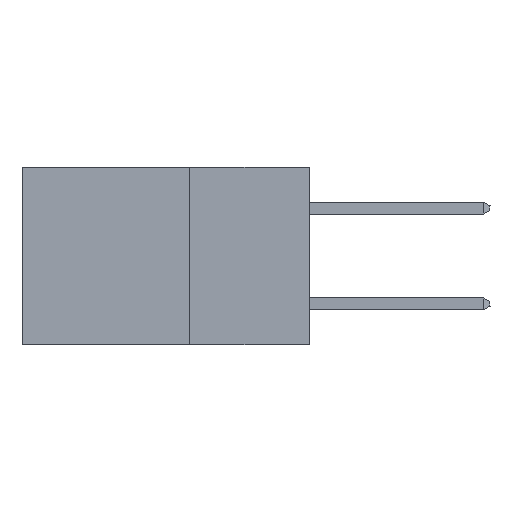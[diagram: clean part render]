
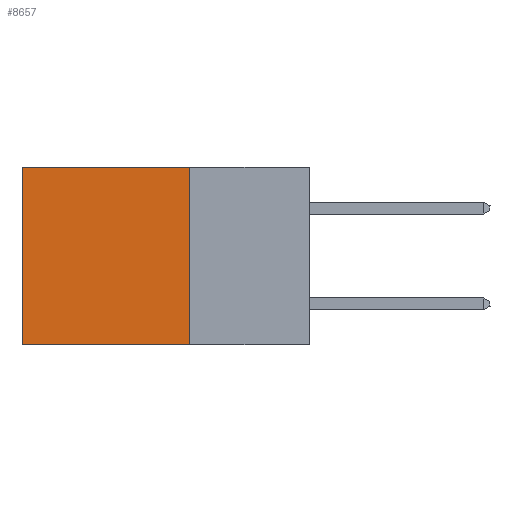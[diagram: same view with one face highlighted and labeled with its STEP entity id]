
A CAD part, left-side view. The second image highlights one B-rep face of the part: STEP entity #8657.
In plain terms, the highlighted planar face has unit normal (-1, 0, 0).
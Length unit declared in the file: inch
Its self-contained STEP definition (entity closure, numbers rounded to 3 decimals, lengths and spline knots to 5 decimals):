
#1060 = DIRECTION ( 'NONE',  ( 0., 1., 0. ) ) ;
#1374 = CARTESIAN_POINT ( 'NONE',  ( 0.2875, 0.25, -0.37 ) ) ;
#1828 = VECTOR ( 'NONE', #12287, 39.37008 ) ;
#1900 = CARTESIAN_POINT ( 'NONE',  ( 0.2875, 0.6, -0.37 ) ) ;
#3026 = CARTESIAN_POINT ( 'NONE',  ( 0.2875, 0.25, 0. ) ) ;
#3926 = VERTEX_POINT ( 'NONE', #17278 ) ;
#4363 = ORIENTED_EDGE ( 'NONE', *, *, #5215, .T. ) ;
#5124 = FACE_OUTER_BOUND ( 'NONE', #15097, .T. ) ;
#5215 = EDGE_CURVE ( 'NONE', #13371, #7720, #6733, .T. ) ;
#5445 = CARTESIAN_POINT ( 'NONE',  ( 0.2875, 0.6, 0. ) ) ;
#5970 = CARTESIAN_POINT ( 'NONE',  ( 0.2875, 0.6, 0. ) ) ;
#6553 = CARTESIAN_POINT ( 'NONE',  ( 0.2875, 0.25, -0.37 ) ) ;
#6733 = LINE ( 'NONE', #5445, #13678 ) ;
#6949 = CARTESIAN_POINT ( 'NONE',  ( 0.2875, 0.25, 0. ) ) ;
#7202 = VECTOR ( 'NONE', #1060, 39.37008 ) ;
#7720 = VERTEX_POINT ( 'NONE', #1900 ) ;
#8106 = VERTEX_POINT ( 'NONE', #1374 ) ;
#8268 = DIRECTION ( 'NONE',  ( 0., 0., -1. ) ) ;
#8657 = ADVANCED_FACE ( 'NONE', ( #5124 ), #14762, .F. ) ;
#9138 = ORIENTED_EDGE ( 'NONE', *, *, #10377, .T. ) ;
#9436 = EDGE_CURVE ( 'NONE', #8106, #7720, #17158, .T. ) ;
#10338 = AXIS2_PLACEMENT_3D ( 'NONE', #6949, #16045, #8268 ) ;
#10377 = EDGE_CURVE ( 'NONE', #3926, #13371, #16341, .T. ) ;
#10893 = DIRECTION ( 'NONE',  ( 0., 0., -1. ) ) ;
#12287 = DIRECTION ( 'NONE',  ( 0., 1., 0. ) ) ;
#13371 = VERTEX_POINT ( 'NONE', #5970 ) ;
#13440 = VECTOR ( 'NONE', #10893, 39.37008 ) ;
#13524 = CARTESIAN_POINT ( 'NONE',  ( 0.2875, 0.25, 0. ) ) ;
#13678 = VECTOR ( 'NONE', #17192, 39.37008 ) ;
#13866 = LINE ( 'NONE', #13524, #13440 ) ;
#14742 = ORIENTED_EDGE ( 'NONE', *, *, #15134, .F. ) ;
#14762 = PLANE ( 'NONE',  #10338 ) ;
#14922 = ORIENTED_EDGE ( 'NONE', *, *, #9436, .F. ) ;
#15097 = EDGE_LOOP ( 'NONE', ( #4363, #14922, #14742, #9138 ) ) ;
#15134 = EDGE_CURVE ( 'NONE', #3926, #8106, #13866, .T. ) ;
#16045 = DIRECTION ( 'NONE',  ( 1., 0., 0. ) ) ;
#16341 = LINE ( 'NONE', #3026, #1828 ) ;
#17158 = LINE ( 'NONE', #6553, #7202 ) ;
#17192 = DIRECTION ( 'NONE',  ( 0., 0., -1. ) ) ;
#17278 = CARTESIAN_POINT ( 'NONE',  ( 0.2875, 0.25, 0. ) ) ;
